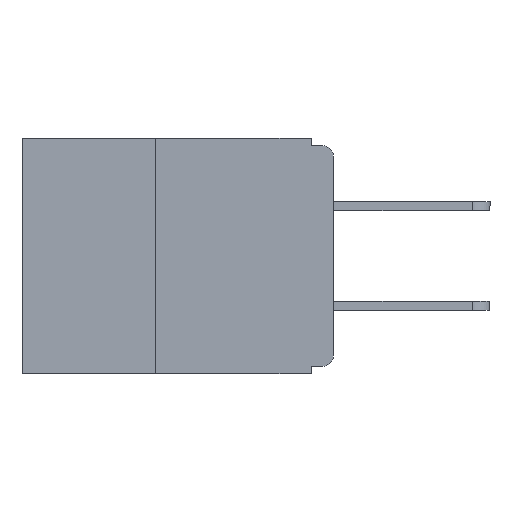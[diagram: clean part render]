
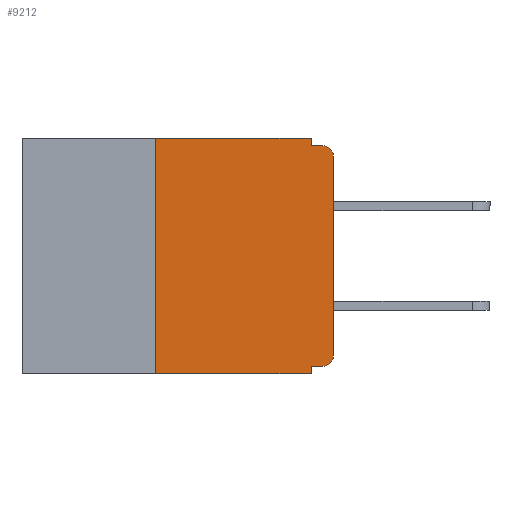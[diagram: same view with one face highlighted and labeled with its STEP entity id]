
A CAD part, left-side view. The second image highlights one B-rep face of the part: STEP entity #9212.
In plain terms, the highlighted planar face has unit normal (-1, 0, 0).
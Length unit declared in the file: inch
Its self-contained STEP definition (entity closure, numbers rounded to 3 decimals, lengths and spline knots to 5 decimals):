
#97 = DIRECTION ( 'NONE',  ( 0., 0., -1. ) ) ;
#139 = CARTESIAN_POINT ( 'NONE',  ( 0., 0.437, 0. ) ) ;
#779 = EDGE_CURVE ( 'NONE', #11897, #1843, #10782, .T. ) ;
#809 = VERTEX_POINT ( 'NONE', #6985 ) ;
#850 = VECTOR ( 'NONE', #5425, 39.37008 ) ;
#894 = CARTESIAN_POINT ( 'NONE',  ( 0., 0.015, -0.305 ) ) ;
#1112 = ORIENTED_EDGE ( 'NONE', *, *, #12362, .F. ) ;
#1166 = LINE ( 'NONE', #12538, #850 ) ;
#1174 = VERTEX_POINT ( 'NONE', #9580 ) ;
#1229 = ORIENTED_EDGE ( 'NONE', *, *, #11255, .F. ) ;
#1330 = DIRECTION ( 'NONE',  ( 0., 1., 0. ) ) ;
#1489 = FACE_OUTER_BOUND ( 'NONE', #4795, .T. ) ;
#1641 = CIRCLE ( 'NONE', #8793, 0.015 ) ;
#1675 = CARTESIAN_POINT ( 'NONE',  ( 0., 0., 0. ) ) ;
#1843 = VERTEX_POINT ( 'NONE', #6785 ) ;
#1906 = DIRECTION ( 'NONE',  ( 0., 0., -1. ) ) ;
#1947 = LINE ( 'NONE', #6417, #4039 ) ;
#2376 = CARTESIAN_POINT ( 'NONE',  ( 0., 0., -0.01 ) ) ;
#2446 = EDGE_CURVE ( 'NONE', #7572, #9379, #9640, .T. ) ;
#2472 = ORIENTED_EDGE ( 'NONE', *, *, #3951, .F. ) ;
#2673 = VECTOR ( 'NONE', #11139, 39.37008 ) ;
#3023 = ORIENTED_EDGE ( 'NONE', *, *, #3497, .T. ) ;
#3147 = DIRECTION ( 'NONE',  ( 0., -1., 0. ) ) ;
#3359 = CARTESIAN_POINT ( 'NONE',  ( 0., 0.25, 0. ) ) ;
#3429 = CARTESIAN_POINT ( 'NONE',  ( 0., 0.015, -0.01 ) ) ;
#3467 = CARTESIAN_POINT ( 'NONE',  ( 0., 0.015, -0.32 ) ) ;
#3497 = EDGE_CURVE ( 'NONE', #809, #7044, #10286, .T. ) ;
#3512 = CARTESIAN_POINT ( 'NONE',  ( 0., 0.031, -0.32 ) ) ;
#3762 = CARTESIAN_POINT ( 'NONE',  ( 0., 0.015, -0.025 ) ) ;
#3863 = ORIENTED_EDGE ( 'NONE', *, *, #6973, .F. ) ;
#3902 = CARTESIAN_POINT ( 'NONE',  ( 0., 0.437, -0.33 ) ) ;
#3951 = EDGE_CURVE ( 'NONE', #9379, #1174, #10574, .T. ) ;
#4039 = VECTOR ( 'NONE', #1330, 39.37008 ) ;
#4142 = CARTESIAN_POINT ( 'NONE',  ( 0., 0.031, 0. ) ) ;
#4146 = VERTEX_POINT ( 'NONE', #3467 ) ;
#4288 = ORIENTED_EDGE ( 'NONE', *, *, #7000, .F. ) ;
#4737 = CARTESIAN_POINT ( 'NONE',  ( 0., 0.25, -0.33 ) ) ;
#4744 = DIRECTION ( 'NONE',  ( 0., 0., -1. ) ) ;
#4773 = DIRECTION ( 'NONE',  ( 0., 0., -1. ) ) ;
#4795 = EDGE_LOOP ( 'NONE', ( #6298, #12984, #4288, #2472, #11007, #1112, #3023, #1229, #3863, #6424 ) ) ;
#4874 = VECTOR ( 'NONE', #4911, 39.37008 ) ;
#4911 = DIRECTION ( 'NONE',  ( 0., -1., 0. ) ) ;
#5425 = DIRECTION ( 'NONE',  ( 0., 0., -1. ) ) ;
#5577 = VERTEX_POINT ( 'NONE', #3429 ) ;
#5716 = CARTESIAN_POINT ( 'NONE',  ( 0., 0.437, 0. ) ) ;
#6298 = ORIENTED_EDGE ( 'NONE', *, *, #779, .T. ) ;
#6417 = CARTESIAN_POINT ( 'NONE',  ( 0., 0., -0.32 ) ) ;
#6424 = ORIENTED_EDGE ( 'NONE', *, *, #11552, .T. ) ;
#6543 = EDGE_CURVE ( 'NONE', #1843, #5577, #1641, .T. ) ;
#6570 = LINE ( 'NONE', #4737, #9578 ) ;
#6728 = DIRECTION ( 'NONE',  ( 0., 0., 1. ) ) ;
#6785 = CARTESIAN_POINT ( 'NONE',  ( 0., 0., -0.025 ) ) ;
#6973 = EDGE_CURVE ( 'NONE', #4146, #7067, #1947, .T. ) ;
#6985 = CARTESIAN_POINT ( 'NONE',  ( 0., 0.25, -0.33 ) ) ;
#7000 = EDGE_CURVE ( 'NONE', #1174, #5577, #11484, .T. ) ;
#7044 = VERTEX_POINT ( 'NONE', #8004 ) ;
#7067 = VERTEX_POINT ( 'NONE', #3512 ) ;
#7572 = VERTEX_POINT ( 'NONE', #3359 ) ;
#7885 = VECTOR ( 'NONE', #97, 39.37008 ) ;
#7886 = AXIS2_PLACEMENT_3D ( 'NONE', #5716, #10809, #4744 ) ;
#8004 = CARTESIAN_POINT ( 'NONE',  ( 0., 0.031, -0.33 ) ) ;
#8009 = DIRECTION ( 'NONE',  ( -1., 0., 0. ) ) ;
#8793 = AXIS2_PLACEMENT_3D ( 'NONE', #3762, #10837, #4773 ) ;
#9212 = ADVANCED_FACE ( 'NONE', ( #1489 ), #11799, .F. ) ;
#9379 = VERTEX_POINT ( 'NONE', #11765 ) ;
#9512 = DIRECTION ( 'NONE',  ( 0., -1., 0. ) ) ;
#9578 = VECTOR ( 'NONE', #6728, 39.37008 ) ;
#9580 = CARTESIAN_POINT ( 'NONE',  ( 0., 0.031, -0.01 ) ) ;
#9640 = LINE ( 'NONE', #139, #12032 ) ;
#9953 = AXIS2_PLACEMENT_3D ( 'NONE', #894, #8009, #1906 ) ;
#10286 = LINE ( 'NONE', #3902, #4874 ) ;
#10574 = LINE ( 'NONE', #4142, #7885 ) ;
#10782 = LINE ( 'NONE', #1675, #2673 ) ;
#10809 = DIRECTION ( 'NONE',  ( 1., 0., 0. ) ) ;
#10837 = DIRECTION ( 'NONE',  ( -1., 0., 0. ) ) ;
#10847 = CIRCLE ( 'NONE', #9953, 0.015 ) ;
#11007 = ORIENTED_EDGE ( 'NONE', *, *, #2446, .F. ) ;
#11139 = DIRECTION ( 'NONE',  ( 0., 0., 1. ) ) ;
#11255 = EDGE_CURVE ( 'NONE', #7067, #7044, #1166, .T. ) ;
#11484 = LINE ( 'NONE', #2376, #11808 ) ;
#11552 = EDGE_CURVE ( 'NONE', #4146, #11897, #10847, .T. ) ;
#11581 = CARTESIAN_POINT ( 'NONE',  ( 0., 0., -0.305 ) ) ;
#11765 = CARTESIAN_POINT ( 'NONE',  ( 0., 0.031, 0. ) ) ;
#11799 = PLANE ( 'NONE',  #7886 ) ;
#11808 = VECTOR ( 'NONE', #9512, 39.37008 ) ;
#11897 = VERTEX_POINT ( 'NONE', #11581 ) ;
#12032 = VECTOR ( 'NONE', #3147, 39.37008 ) ;
#12362 = EDGE_CURVE ( 'NONE', #809, #7572, #6570, .T. ) ;
#12538 = CARTESIAN_POINT ( 'NONE',  ( 0., 0.031, -0.33 ) ) ;
#12984 = ORIENTED_EDGE ( 'NONE', *, *, #6543, .T. ) ;
